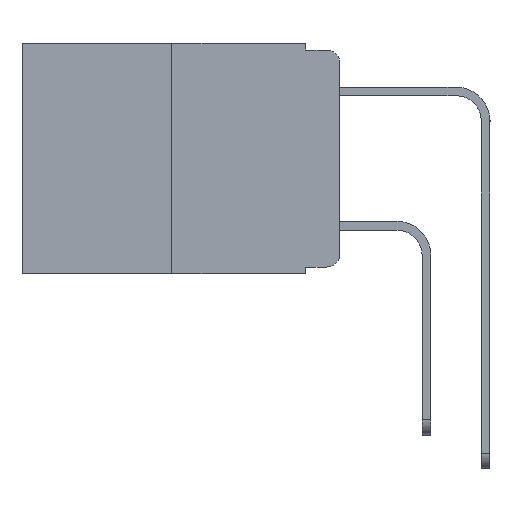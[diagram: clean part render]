
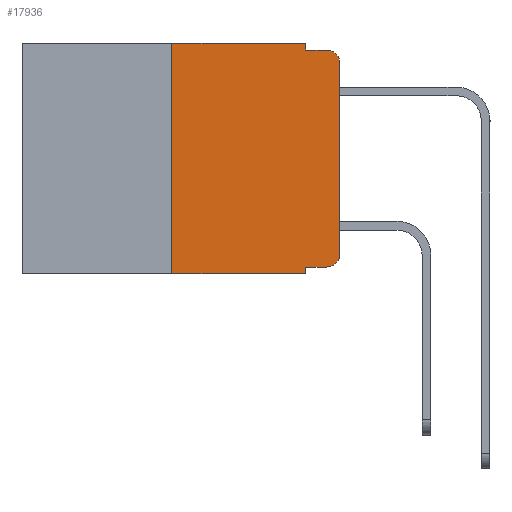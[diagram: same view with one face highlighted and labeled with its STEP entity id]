
A CAD part, left-side view. The second image highlights one B-rep face of the part: STEP entity #17936.
In plain terms, the highlighted planar face has unit normal (-1, 0, 0).
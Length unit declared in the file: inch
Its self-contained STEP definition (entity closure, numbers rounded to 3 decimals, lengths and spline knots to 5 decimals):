
#650 = EDGE_CURVE ( 'NONE', #8191, #5165, #15332, .T. ) ;
#1311 = AXIS2_PLACEMENT_3D ( 'NONE', #15805, #5602, #17486 ) ;
#1467 = VERTEX_POINT ( 'NONE', #10944 ) ;
#1758 = EDGE_CURVE ( 'NONE', #11157, #18267, #2147, .T. ) ;
#2071 = DIRECTION ( 'NONE',  ( -1., 0., 0. ) ) ;
#2147 = LINE ( 'NONE', #6356, #11251 ) ;
#2414 = VECTOR ( 'NONE', #21837, 39.37008 ) ;
#2488 = CARTESIAN_POINT ( 'NONE',  ( 0., 0.051, 0. ) ) ;
#2890 = AXIS2_PLACEMENT_3D ( 'NONE', #9558, #21326, #11284 ) ;
#3087 = CIRCLE ( 'NONE', #1311, 0.02 ) ;
#3146 = ORIENTED_EDGE ( 'NONE', *, *, #5250, .T. ) ;
#3432 = ORIENTED_EDGE ( 'NONE', *, *, #15763, .F. ) ;
#3656 = LINE ( 'NONE', #8114, #7636 ) ;
#3810 = VECTOR ( 'NONE', #14458, 39.37008 ) ;
#4181 = DIRECTION ( 'NONE',  ( 0., -1., 0. ) ) ;
#4648 = DIRECTION ( 'NONE',  ( 0., 0., -1. ) ) ;
#5165 = VERTEX_POINT ( 'NONE', #16362 ) ;
#5250 = EDGE_CURVE ( 'NONE', #5165, #1467, #6398, .T. ) ;
#5330 = ORIENTED_EDGE ( 'NONE', *, *, #11389, .F. ) ;
#5417 = DIRECTION ( 'NONE',  ( 0., 0., -1. ) ) ;
#5602 = DIRECTION ( 'NONE',  ( -1., 0., 0. ) ) ;
#6064 = AXIS2_PLACEMENT_3D ( 'NONE', #16798, #2071, #4648 ) ;
#6151 = VECTOR ( 'NONE', #4181, 39.37008 ) ;
#6356 = CARTESIAN_POINT ( 'NONE',  ( 0., 0.25, 0. ) ) ;
#6398 = LINE ( 'NONE', #18252, #10416 ) ;
#6456 = LINE ( 'NONE', #8868, #19974 ) ;
#6959 = LINE ( 'NONE', #20212, #2414 ) ;
#6985 = CARTESIAN_POINT ( 'NONE',  ( 0., 0.25, -0.343 ) ) ;
#7295 = CARTESIAN_POINT ( 'NONE',  ( 0., 0.051, -0.343 ) ) ;
#7636 = VECTOR ( 'NONE', #21589, 39.37008 ) ;
#8114 = CARTESIAN_POINT ( 'NONE',  ( 0., 0.473, 0. ) ) ;
#8191 = VERTEX_POINT ( 'NONE', #14748 ) ;
#8868 = CARTESIAN_POINT ( 'NONE',  ( 0., 0.051, -0.01 ) ) ;
#9438 = ORIENTED_EDGE ( 'NONE', *, *, #650, .T. ) ;
#9558 = CARTESIAN_POINT ( 'NONE',  ( 0., 0.473, 0. ) ) ;
#9668 = VERTEX_POINT ( 'NONE', #19625 ) ;
#9950 = FACE_OUTER_BOUND ( 'NONE', #11952, .T. ) ;
#10211 = VERTEX_POINT ( 'NONE', #17644 ) ;
#10416 = VECTOR ( 'NONE', #11519, 39.37008 ) ;
#10658 = CARTESIAN_POINT ( 'NONE',  ( 0., 0.051, 0. ) ) ;
#10689 = LINE ( 'NONE', #10965, #6151 ) ;
#10944 = CARTESIAN_POINT ( 'NONE',  ( 0., 0., -0.03 ) ) ;
#10965 = CARTESIAN_POINT ( 'NONE',  ( 0., 0.473, -0.343 ) ) ;
#11157 = VERTEX_POINT ( 'NONE', #6985 ) ;
#11251 = VECTOR ( 'NONE', #18236, 39.37008 ) ;
#11284 = DIRECTION ( 'NONE',  ( 0., 0., -1. ) ) ;
#11389 = EDGE_CURVE ( 'NONE', #16130, #10211, #21246, .T. ) ;
#11519 = DIRECTION ( 'NONE',  ( 0., 0., 1. ) ) ;
#11536 = LINE ( 'NONE', #15612, #20480 ) ;
#11616 = ORIENTED_EDGE ( 'NONE', *, *, #18279, .F. ) ;
#11715 = VERTEX_POINT ( 'NONE', #16885 ) ;
#11952 = EDGE_LOOP ( 'NONE', ( #3146, #17281, #18318, #5330, #3432, #13058, #15629, #11616, #21067, #9438 ) ) ;
#13058 = ORIENTED_EDGE ( 'NONE', *, *, #1758, .F. ) ;
#13978 = VERTEX_POINT ( 'NONE', #7295 ) ;
#14059 = EDGE_CURVE ( 'NONE', #11157, #13978, #10689, .T. ) ;
#14458 = DIRECTION ( 'NONE',  ( 0., 0., -1. ) ) ;
#14748 = CARTESIAN_POINT ( 'NONE',  ( 0., 0.02, -0.333 ) ) ;
#15332 = CIRCLE ( 'NONE', #6064, 0.02 ) ;
#15542 = CARTESIAN_POINT ( 'NONE',  ( 0., 0.25, 0. ) ) ;
#15612 = CARTESIAN_POINT ( 'NONE',  ( 0., 0.051, 0. ) ) ;
#15629 = ORIENTED_EDGE ( 'NONE', *, *, #14059, .T. ) ;
#15763 = EDGE_CURVE ( 'NONE', #18267, #16130, #3656, .T. ) ;
#15805 = CARTESIAN_POINT ( 'NONE',  ( 0., 0.02, -0.03 ) ) ;
#16106 = EDGE_CURVE ( 'NONE', #1467, #11715, #3087, .T. ) ;
#16130 = VERTEX_POINT ( 'NONE', #10658 ) ;
#16355 = PLANE ( 'NONE',  #2890 ) ;
#16362 = CARTESIAN_POINT ( 'NONE',  ( 0., 0., -0.313 ) ) ;
#16798 = CARTESIAN_POINT ( 'NONE',  ( 0., 0.02, -0.313 ) ) ;
#16885 = CARTESIAN_POINT ( 'NONE',  ( 0., 0.02, -0.01 ) ) ;
#17281 = ORIENTED_EDGE ( 'NONE', *, *, #16106, .T. ) ;
#17486 = DIRECTION ( 'NONE',  ( 0., 0., -1. ) ) ;
#17644 = CARTESIAN_POINT ( 'NONE',  ( 0., 0.051, -0.01 ) ) ;
#17936 = ADVANCED_FACE ( 'NONE', ( #9950 ), #16355, .F. ) ;
#18236 = DIRECTION ( 'NONE',  ( 0., 0., 1. ) ) ;
#18252 = CARTESIAN_POINT ( 'NONE',  ( 0., 0., 0. ) ) ;
#18267 = VERTEX_POINT ( 'NONE', #15542 ) ;
#18279 = EDGE_CURVE ( 'NONE', #9668, #13978, #11536, .T. ) ;
#18318 = ORIENTED_EDGE ( 'NONE', *, *, #18331, .F. ) ;
#18331 = EDGE_CURVE ( 'NONE', #10211, #11715, #6456, .T. ) ;
#19392 = EDGE_CURVE ( 'NONE', #9668, #8191, #6959, .T. ) ;
#19625 = CARTESIAN_POINT ( 'NONE',  ( 0., 0.051, -0.333 ) ) ;
#19974 = VECTOR ( 'NONE', #20692, 39.37008 ) ;
#20212 = CARTESIAN_POINT ( 'NONE',  ( 0., 0.051, -0.333 ) ) ;
#20480 = VECTOR ( 'NONE', #5417, 39.37008 ) ;
#20692 = DIRECTION ( 'NONE',  ( 0., -1., 0. ) ) ;
#21067 = ORIENTED_EDGE ( 'NONE', *, *, #19392, .T. ) ;
#21246 = LINE ( 'NONE', #2488, #3810 ) ;
#21326 = DIRECTION ( 'NONE',  ( 1., 0., 0. ) ) ;
#21589 = DIRECTION ( 'NONE',  ( 0., -1., 0. ) ) ;
#21837 = DIRECTION ( 'NONE',  ( 0., -1., 0. ) ) ;
